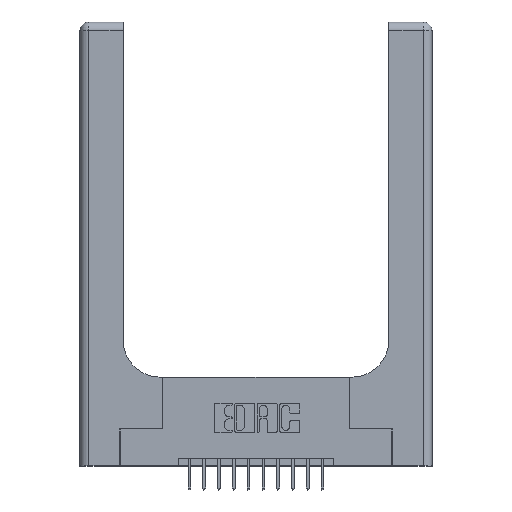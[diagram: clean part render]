
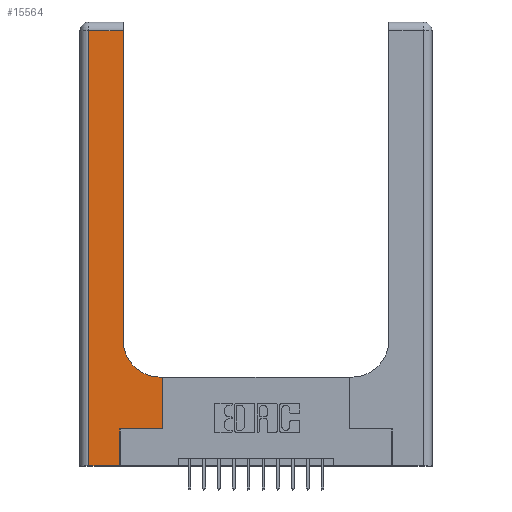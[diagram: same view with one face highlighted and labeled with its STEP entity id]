
A CAD part, top view. The second image highlights one B-rep face of the part: STEP entity #15564.
In plain terms, the highlighted planar face has unit normal (0, 0, 1).
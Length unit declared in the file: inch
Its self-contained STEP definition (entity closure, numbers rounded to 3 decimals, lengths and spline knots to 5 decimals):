
#424 = LINE ( 'NONE', #7380, #15321 ) ;
#687 = PLANE ( 'NONE',  #5014 ) ;
#843 = DIRECTION ( 'NONE',  ( -1., 0., 0. ) ) ;
#873 = VERTEX_POINT ( 'NONE', #7242 ) ;
#913 = VERTEX_POINT ( 'NONE', #1635 ) ;
#1070 = LINE ( 'NONE', #14287, #2127 ) ;
#1313 = EDGE_CURVE ( 'NONE', #15147, #7278, #1070, .T. ) ;
#1588 = ORIENTED_EDGE ( 'NONE', *, *, #14598, .T. ) ;
#1635 = CARTESIAN_POINT ( 'NONE',  ( 0.2915, 0.85, 0.37 ) ) ;
#1701 = EDGE_CURVE ( 'NONE', #873, #913, #4444, .T. ) ;
#1868 = VERTEX_POINT ( 'NONE', #3027 ) ;
#2127 = VECTOR ( 'NONE', #7499, 39.37008 ) ;
#2402 = VECTOR ( 'NONE', #8843, 39.37008 ) ;
#3027 = CARTESIAN_POINT ( 'NONE',  ( 0.5585, 0.6, 0.37 ) ) ;
#3443 = EDGE_CURVE ( 'NONE', #7278, #7219, #6527, .T. ) ;
#3710 = CARTESIAN_POINT ( 'NONE',  ( 0., 2.94, 0.37 ) ) ;
#3933 = VECTOR ( 'NONE', #6595, 39.37008 ) ;
#3988 = AXIS2_PLACEMENT_3D ( 'NONE', #5513, #12210, #16020 ) ;
#4072 = LINE ( 'NONE', #3710, #12201 ) ;
#4255 = ORIENTED_EDGE ( 'NONE', *, *, #3443, .T. ) ;
#4444 = CIRCLE ( 'NONE', #3988, 0.25 ) ;
#5014 = AXIS2_PLACEMENT_3D ( 'NONE', #8379, #12740, #843 ) ;
#5223 = CARTESIAN_POINT ( 'NONE',  ( 0.5585, 0.25, 0.37 ) ) ;
#5374 = ORIENTED_EDGE ( 'NONE', *, *, #9939, .T. ) ;
#5379 = LINE ( 'NONE', #10513, #17363 ) ;
#5445 = ORIENTED_EDGE ( 'NONE', *, *, #1701, .T. ) ;
#5513 = CARTESIAN_POINT ( 'NONE',  ( 0.5415, 0.85, 0.37 ) ) ;
#5687 = ORIENTED_EDGE ( 'NONE', *, *, #13193, .T. ) ;
#5708 = EDGE_CURVE ( 'NONE', #913, #13019, #11020, .T. ) ;
#6036 = DIRECTION ( 'NONE',  ( 1., 0., 0. ) ) ;
#6061 = DIRECTION ( 'NONE',  ( 1., 0., 0. ) ) ;
#6229 = LINE ( 'NONE', #5223, #3933 ) ;
#6527 = LINE ( 'NONE', #7306, #13247 ) ;
#6595 = DIRECTION ( 'NONE',  ( 0., 1., 0. ) ) ;
#6673 = ORIENTED_EDGE ( 'NONE', *, *, #5708, .T. ) ;
#7219 = VERTEX_POINT ( 'NONE', #15053 ) ;
#7242 = CARTESIAN_POINT ( 'NONE',  ( 0.5415, 0.6, 0.37 ) ) ;
#7278 = VERTEX_POINT ( 'NONE', #9118 ) ;
#7306 = CARTESIAN_POINT ( 'NONE',  ( 0., 0., 0.37 ) ) ;
#7380 = CARTESIAN_POINT ( 'NONE',  ( 0.269, 0.25, 0.37 ) ) ;
#7499 = DIRECTION ( 'NONE',  ( 0., -1., 0. ) ) ;
#7870 = ORIENTED_EDGE ( 'NONE', *, *, #12118, .T. ) ;
#7950 = ORIENTED_EDGE ( 'NONE', *, *, #13477, .T. ) ;
#8379 = CARTESIAN_POINT ( 'NONE',  ( 0., 3., 0.37 ) ) ;
#8664 = CARTESIAN_POINT ( 'NONE',  ( 0.2915, 0.6, 0.37 ) ) ;
#8705 = LINE ( 'NONE', #8664, #2402 ) ;
#8843 = DIRECTION ( 'NONE',  ( -1., 0., 0. ) ) ;
#9118 = CARTESIAN_POINT ( 'NONE',  ( 0.06, 0., 0.37 ) ) ;
#9200 = DIRECTION ( 'NONE',  ( -1., 0., 0. ) ) ;
#9939 = EDGE_CURVE ( 'NONE', #12741, #10063, #424, .T. ) ;
#10063 = VERTEX_POINT ( 'NONE', #13657 ) ;
#10310 = EDGE_LOOP ( 'NONE', ( #6673, #1588, #10676, #4255, #7950, #5374, #7870, #5687, #5445 ) ) ;
#10513 = CARTESIAN_POINT ( 'NONE',  ( 0.269, 0., 0.37 ) ) ;
#10676 = ORIENTED_EDGE ( 'NONE', *, *, #1313, .T. ) ;
#10897 = FACE_OUTER_BOUND ( 'NONE', #10310, .T. ) ;
#11020 = LINE ( 'NONE', #14317, #13580 ) ;
#11040 = CARTESIAN_POINT ( 'NONE',  ( 0.2915, 2.94, 0.37 ) ) ;
#11711 = CARTESIAN_POINT ( 'NONE',  ( 0.269, 0.25, 0.37 ) ) ;
#12118 = EDGE_CURVE ( 'NONE', #10063, #1868, #6229, .T. ) ;
#12201 = VECTOR ( 'NONE', #9200, 39.37008 ) ;
#12210 = DIRECTION ( 'NONE',  ( 0., 0., -1. ) ) ;
#12740 = DIRECTION ( 'NONE',  ( 0., 0., -1. ) ) ;
#12741 = VERTEX_POINT ( 'NONE', #11711 ) ;
#12919 = DIRECTION ( 'NONE',  ( 0., 1., 0. ) ) ;
#13019 = VERTEX_POINT ( 'NONE', #11040 ) ;
#13193 = EDGE_CURVE ( 'NONE', #1868, #873, #8705, .T. ) ;
#13247 = VECTOR ( 'NONE', #6036, 39.37008 ) ;
#13477 = EDGE_CURVE ( 'NONE', #7219, #12741, #5379, .T. ) ;
#13580 = VECTOR ( 'NONE', #12919, 39.37008 ) ;
#13657 = CARTESIAN_POINT ( 'NONE',  ( 0.5585, 0.25, 0.37 ) ) ;
#14287 = CARTESIAN_POINT ( 'NONE',  ( 0.06, 3., 0.37 ) ) ;
#14317 = CARTESIAN_POINT ( 'NONE',  ( 0.2915, 3., 0.37 ) ) ;
#14598 = EDGE_CURVE ( 'NONE', #13019, #15147, #4072, .T. ) ;
#14685 = DIRECTION ( 'NONE',  ( 0., 1., 0. ) ) ;
#15053 = CARTESIAN_POINT ( 'NONE',  ( 0.269, 0., 0.37 ) ) ;
#15147 = VERTEX_POINT ( 'NONE', #16082 ) ;
#15321 = VECTOR ( 'NONE', #6061, 39.37008 ) ;
#15564 = ADVANCED_FACE ( 'NONE', ( #10897 ), #687, .F. ) ;
#16020 = DIRECTION ( 'NONE',  ( 1., 0., 0. ) ) ;
#16082 = CARTESIAN_POINT ( 'NONE',  ( 0.06, 2.94, 0.37 ) ) ;
#17363 = VECTOR ( 'NONE', #14685, 39.37008 ) ;
